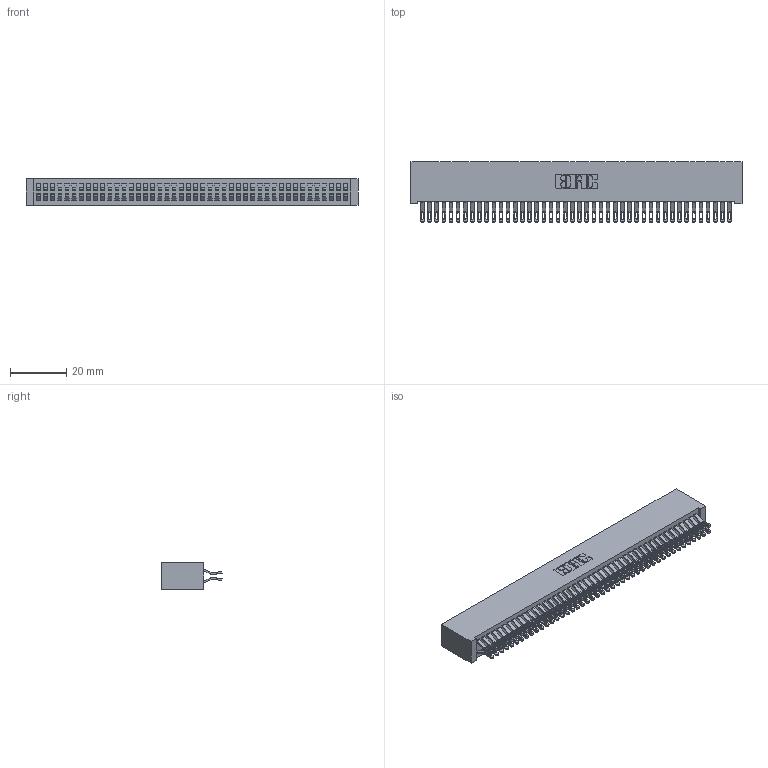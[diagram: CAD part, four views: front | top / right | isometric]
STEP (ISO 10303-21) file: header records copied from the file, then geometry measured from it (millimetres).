
FILE_DESCRIPTION (( 'STEP AP203' ), '1' );
FILE_NAME ('342-088-555-201.STEP', '2018-08-13T20:53:21', ( '' ), ( '' ), 'SwSTEP 2.0', 'SolidWorks 2016', '' );
FILE_SCHEMA (( 'CONFIG_CONTROL_DESIGN' ));
Length unit declared in the file: inch
Products named in the file (3): 345-292-001_555 Tail; 342-088-555-201; 342 Part_Lugless
Assembly tree (89 placements, depth 2):
  342-088-555-201
    342 Part_Lugless
    345-292-001_555 Tail  x88
Bounding box: 118.01 x 21.47 x 9.4 mm (x, y, z)
Volume: 11296.6 mm3; surface area: 19734.9 mm2
Topology: 89 solids, 89 shells, 5206 faces, 16379 edges, 10918 vertices
Faces by surface type: plane 3054, cylinder 2152
Entity records: 27965 total; most frequent: CARTESIAN_POINT 4664, ORIENTED_EDGE 4570, DIRECTION 3945, EDGE_CURVE 2285, VECTOR 2145, LINE 2145, VERTEX_POINT 1522, AXIS2_PLACEMENT_3D 900
